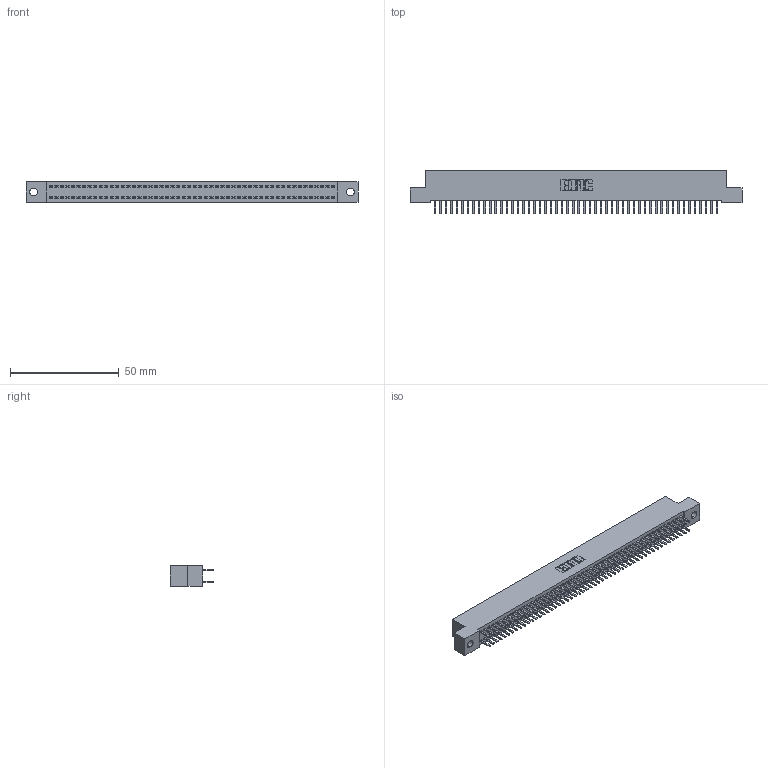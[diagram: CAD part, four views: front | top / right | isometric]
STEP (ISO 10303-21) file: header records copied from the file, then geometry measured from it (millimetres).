
FILE_DESCRIPTION (( 'STEP AP203' ), '1' );
FILE_NAME ('392-104-520-202.STEP', '2019-10-09T21:45:44', ( '' ), ( '' ), 'SwSTEP 2.0', 'SolidWorks 2016', '' );
FILE_SCHEMA (( 'CONFIG_CONTROL_DESIGN' ));
Length unit declared in the file: inch
Products named in the file (3): 342 Part_.128 Slot; 345-292-001_345-293-120; 392-104-520-202
Assembly tree (105 placements, depth 2):
  392-104-520-202
    342 Part_.128 Slot
    345-292-001_345-293-120  x104
Bounding box: 152.4 x 20.02 x 9.4 mm (x, y, z)
Volume: 13642.6 mm3; surface area: 22104.7 mm2
Topology: 105 solids, 105 shells, 5938 faces, 17263 edges, 11230 vertices
Faces by surface type: plane 4022, cylinder 1916
Entity records: 32277 total; most frequent: CARTESIAN_POINT 5350, ORIENTED_EDGE 5274, DIRECTION 4541, EDGE_CURVE 2637, VECTOR 2505, LINE 2505, VERTEX_POINT 1754, AXIS2_PLACEMENT_3D 1018
